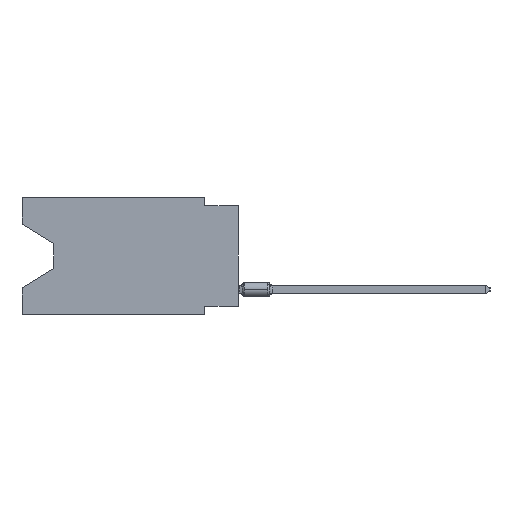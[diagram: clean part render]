
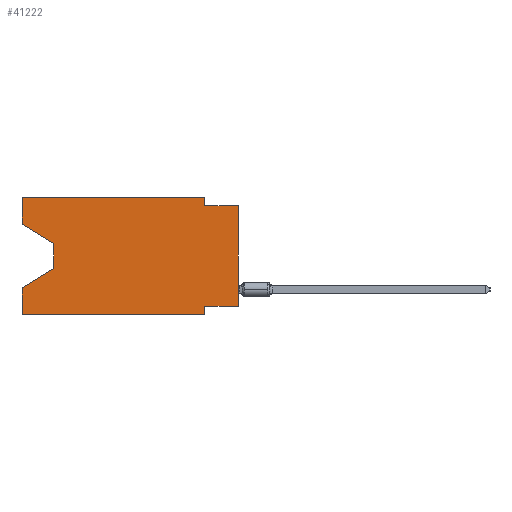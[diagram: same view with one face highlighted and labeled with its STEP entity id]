
A CAD part, left-side view. The second image highlights one B-rep face of the part: STEP entity #41222.
In plain terms, the highlighted planar face has unit normal (-1, 0, 0).
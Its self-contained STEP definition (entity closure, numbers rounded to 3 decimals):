
#195 = VECTOR ( 'NONE', #28258, 1000. ) ;
#624 = LINE ( 'NONE', #41569, #5581 ) ;
#747 = VERTEX_POINT ( 'NONE', #25045 ) ;
#1102 = DIRECTION ( 'NONE',  ( 0., 0.855, -0.519 ) ) ;
#1442 = DIRECTION ( 'NONE',  ( 0., -0.855, -0.519 ) ) ;
#1961 = EDGE_CURVE ( 'NONE', #39290, #53400, #624, .T. ) ;
#2224 = CARTESIAN_POINT ( 'NONE',  ( 0., 16.383, -2.038 ) ) ;
#2319 = DIRECTION ( 'NONE',  ( 0., 0., 1. ) ) ;
#2976 = CARTESIAN_POINT ( 'NONE',  ( 0., 0., 0. ) ) ;
#3018 = PLANE ( 'NONE',  #51827 ) ;
#3379 = CARTESIAN_POINT ( 'NONE',  ( 0., 0., -0.635 ) ) ;
#3583 = LINE ( 'NONE', #33491, #22437 ) ;
#4015 = LINE ( 'NONE', #14426, #4864 ) ;
#4107 = EDGE_CURVE ( 'NONE', #25438, #40284, #4015, .T. ) ;
#4864 = VECTOR ( 'NONE', #55667, 1000. ) ;
#4895 = EDGE_CURVE ( 'NONE', #747, #35484, #7908, .T. ) ;
#5581 = VECTOR ( 'NONE', #46928, 1000. ) ;
#6075 = VERTEX_POINT ( 'NONE', #30632 ) ;
#7041 = LINE ( 'NONE', #2976, #7164 ) ;
#7125 = LINE ( 'NONE', #46415, #66329 ) ;
#7164 = VECTOR ( 'NONE', #2319, 1000. ) ;
#7908 = LINE ( 'NONE', #28742, #42488 ) ;
#9183 = CARTESIAN_POINT ( 'NONE',  ( 0., 13.97, -3.505 ) ) ;
#10788 = ORIENTED_EDGE ( 'NONE', *, *, #52050, .F. ) ;
#12361 = ORIENTED_EDGE ( 'NONE', *, *, #17200, .T. ) ;
#12583 = VERTEX_POINT ( 'NONE', #51945 ) ;
#13402 = CARTESIAN_POINT ( 'NONE',  ( 0., 2.54, -8.255 ) ) ;
#13727 = EDGE_CURVE ( 'NONE', #60729, #25438, #3583, .T. ) ;
#14252 = CARTESIAN_POINT ( 'NONE',  ( 0., 0., -0.635 ) ) ;
#14426 = CARTESIAN_POINT ( 'NONE',  ( 0., 2.54, 0. ) ) ;
#16776 = EDGE_CURVE ( 'NONE', #12583, #6075, #7125, .T. ) ;
#16813 = ORIENTED_EDGE ( 'NONE', *, *, #4107, .F. ) ;
#16855 = CARTESIAN_POINT ( 'NONE',  ( 0., 16.383, 0. ) ) ;
#17200 = EDGE_CURVE ( 'NONE', #42190, #61051, #52766, .T. ) ;
#17871 = EDGE_CURVE ( 'NONE', #39290, #6075, #28863, .T. ) ;
#18136 = DIRECTION ( 'NONE',  ( 0., 0., -1. ) ) ;
#18330 = ORIENTED_EDGE ( 'NONE', *, *, #1961, .T. ) ;
#18505 = LINE ( 'NONE', #3379, #195 ) ;
#22437 = VECTOR ( 'NONE', #44533, 1000. ) ;
#22805 = CARTESIAN_POINT ( 'NONE',  ( 0., 2.54, -8.89 ) ) ;
#23526 = DIRECTION ( 'NONE',  ( 1., 0., 0. ) ) ;
#23988 = LINE ( 'NONE', #9183, #50353 ) ;
#25045 = CARTESIAN_POINT ( 'NONE',  ( 0., 0., -8.255 ) ) ;
#25438 = VERTEX_POINT ( 'NONE', #50603 ) ;
#25895 = VECTOR ( 'NONE', #65393, 1000. ) ;
#28258 = DIRECTION ( 'NONE',  ( 0., -1., 0. ) ) ;
#28742 = CARTESIAN_POINT ( 'NONE',  ( 0., 0., -8.255 ) ) ;
#28863 = LINE ( 'NONE', #35196, #25895 ) ;
#29828 = ORIENTED_EDGE ( 'NONE', *, *, #44687, .T. ) ;
#30632 = CARTESIAN_POINT ( 'NONE',  ( 0., 16.383, -6.852 ) ) ;
#32221 = DIRECTION ( 'NONE',  ( 0., 0., -1. ) ) ;
#33274 = VECTOR ( 'NONE', #1442, 1000. ) ;
#33491 = CARTESIAN_POINT ( 'NONE',  ( 0., 16.383, 0. ) ) ;
#34430 = DIRECTION ( 'NONE',  ( 0., 1., 0. ) ) ;
#34938 = VECTOR ( 'NONE', #63478, 1000. ) ;
#35196 = CARTESIAN_POINT ( 'NONE',  ( 0., 16.383, 0. ) ) ;
#35484 = VERTEX_POINT ( 'NONE', #13402 ) ;
#38941 = FACE_OUTER_BOUND ( 'NONE', #64970, .T. ) ;
#39290 = VERTEX_POINT ( 'NONE', #46835 ) ;
#40284 = VERTEX_POINT ( 'NONE', #66375 ) ;
#41222 = ADVANCED_FACE ( 'NONE', ( #38941 ), #3018, .F. ) ;
#41569 = CARTESIAN_POINT ( 'NONE',  ( 0., 16.383, -8.89 ) ) ;
#41691 = ORIENTED_EDGE ( 'NONE', *, *, #16776, .T. ) ;
#42190 = VERTEX_POINT ( 'NONE', #2224 ) ;
#42488 = VECTOR ( 'NONE', #34430, 1000. ) ;
#43021 = CARTESIAN_POINT ( 'NONE',  ( 0., 16.383, 0. ) ) ;
#43038 = EDGE_CURVE ( 'NONE', #42190, #60729, #63802, .T. ) ;
#44533 = DIRECTION ( 'NONE',  ( 0., -1., 0. ) ) ;
#44687 = EDGE_CURVE ( 'NONE', #747, #53957, #7041, .T. ) ;
#46415 = CARTESIAN_POINT ( 'NONE',  ( 0., 13.97, -5.385 ) ) ;
#46835 = CARTESIAN_POINT ( 'NONE',  ( 0., 16.383, -8.89 ) ) ;
#46928 = DIRECTION ( 'NONE',  ( 0., -1., 0. ) ) ;
#48331 = CARTESIAN_POINT ( 'NONE',  ( 0., 16.383, 0. ) ) ;
#49637 = ORIENTED_EDGE ( 'NONE', *, *, #61073, .F. ) ;
#49858 = EDGE_CURVE ( 'NONE', #61051, #12583, #23988, .T. ) ;
#50353 = VECTOR ( 'NONE', #54475, 1000. ) ;
#50603 = CARTESIAN_POINT ( 'NONE',  ( 0., 2.54, 0. ) ) ;
#51827 = AXIS2_PLACEMENT_3D ( 'NONE', #48331, #23526, #18136 ) ;
#51945 = CARTESIAN_POINT ( 'NONE',  ( 0., 13.97, -5.385 ) ) ;
#52050 = EDGE_CURVE ( 'NONE', #40284, #53957, #18505, .T. ) ;
#52766 = LINE ( 'NONE', #62839, #33274 ) ;
#53299 = LINE ( 'NONE', #22805, #60475 ) ;
#53400 = VERTEX_POINT ( 'NONE', #59409 ) ;
#53957 = VERTEX_POINT ( 'NONE', #14252 ) ;
#54475 = DIRECTION ( 'NONE',  ( 0., 0., -1. ) ) ;
#55667 = DIRECTION ( 'NONE',  ( 0., 0., -1. ) ) ;
#56996 = ORIENTED_EDGE ( 'NONE', *, *, #43038, .F. ) ;
#58330 = ORIENTED_EDGE ( 'NONE', *, *, #17871, .F. ) ;
#59409 = CARTESIAN_POINT ( 'NONE',  ( 0., 2.54, -8.89 ) ) ;
#60475 = VECTOR ( 'NONE', #32221, 1000. ) ;
#60729 = VERTEX_POINT ( 'NONE', #16855 ) ;
#61051 = VERTEX_POINT ( 'NONE', #62057 ) ;
#61073 = EDGE_CURVE ( 'NONE', #35484, #53400, #53299, .T. ) ;
#61387 = ORIENTED_EDGE ( 'NONE', *, *, #49858, .T. ) ;
#61463 = ORIENTED_EDGE ( 'NONE', *, *, #13727, .F. ) ;
#62057 = CARTESIAN_POINT ( 'NONE',  ( 0., 13.97, -3.505 ) ) ;
#62839 = CARTESIAN_POINT ( 'NONE',  ( 0., 16.383, -2.038 ) ) ;
#63478 = DIRECTION ( 'NONE',  ( 0., 0., 1. ) ) ;
#63802 = LINE ( 'NONE', #43021, #34938 ) ;
#63869 = ORIENTED_EDGE ( 'NONE', *, *, #4895, .F. ) ;
#64970 = EDGE_LOOP ( 'NONE', ( #12361, #61387, #41691, #58330, #18330, #49637, #63869, #29828, #10788, #16813, #61463, #56996 ) ) ;
#65393 = DIRECTION ( 'NONE',  ( 0., 0., 1. ) ) ;
#66329 = VECTOR ( 'NONE', #1102, 1000. ) ;
#66375 = CARTESIAN_POINT ( 'NONE',  ( 0., 2.54, -0.635 ) ) ;
